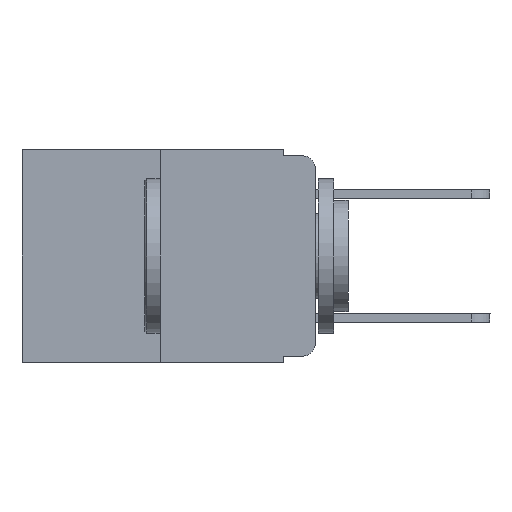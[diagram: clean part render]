
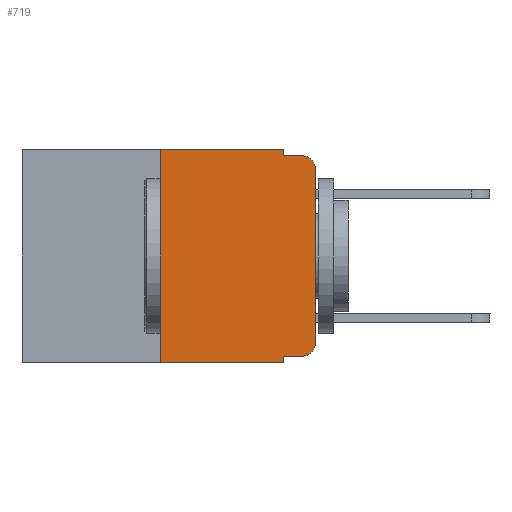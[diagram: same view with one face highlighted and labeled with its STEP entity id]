
A CAD part, left-side view. The second image highlights one B-rep face of the part: STEP entity #719.
In plain terms, the highlighted planar face has unit normal (-1, 0, 0).
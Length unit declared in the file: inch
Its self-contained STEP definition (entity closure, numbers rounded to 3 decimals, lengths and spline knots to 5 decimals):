
#53 = DIRECTION ( 'NONE',  ( 0., -1., 0. ) ) ;
#336 = ORIENTED_EDGE ( 'NONE', *, *, #405, .T. ) ;
#405 = EDGE_CURVE ( 'NONE', #3008, #11672, #10132, .T. ) ;
#460 = DIRECTION ( 'NONE',  ( 1., 0., 0. ) ) ;
#622 = LINE ( 'NONE', #12694, #4878 ) ;
#719 = ADVANCED_FACE ( 'NONE', ( #5134 ), #4983, .F. ) ;
#853 = EDGE_LOOP ( 'NONE', ( #336, #5707, #4773, #11057, #8538, #11031, #7886, #1759, #9447, #5569 ) ) ;
#878 = LINE ( 'NONE', #13318, #14174 ) ;
#914 = CARTESIAN_POINT ( 'NONE',  ( 0., 0.25, -0.343 ) ) ;
#939 = EDGE_CURVE ( 'NONE', #11672, #1989, #8153, .T. ) ;
#1031 = CARTESIAN_POINT ( 'NONE',  ( 0., 0.02, -0.01 ) ) ;
#1291 = CARTESIAN_POINT ( 'NONE',  ( 0., 0.473, -0.343 ) ) ;
#1348 = DIRECTION ( 'NONE',  ( 0., 0., -1. ) ) ;
#1683 = CARTESIAN_POINT ( 'NONE',  ( 0., 0., 0. ) ) ;
#1759 = ORIENTED_EDGE ( 'NONE', *, *, #8592, .F. ) ;
#1989 = VERTEX_POINT ( 'NONE', #1031 ) ;
#2348 = CARTESIAN_POINT ( 'NONE',  ( 0., 0.051, -0.333 ) ) ;
#2366 = LINE ( 'NONE', #1291, #10726 ) ;
#2584 = CARTESIAN_POINT ( 'NONE',  ( 0., 0.051, 0. ) ) ;
#2849 = VERTEX_POINT ( 'NONE', #11474 ) ;
#3008 = VERTEX_POINT ( 'NONE', #6712 ) ;
#3200 = VERTEX_POINT ( 'NONE', #914 ) ;
#3328 = EDGE_CURVE ( 'NONE', #3200, #8352, #622, .T. ) ;
#3452 = LINE ( 'NONE', #9062, #9283 ) ;
#3486 = CARTESIAN_POINT ( 'NONE',  ( 0., 0.02, -0.313 ) ) ;
#3777 = EDGE_CURVE ( 'NONE', #6651, #10921, #3452, .T. ) ;
#3919 = VECTOR ( 'NONE', #11880, 39.37008 ) ;
#3969 = CARTESIAN_POINT ( 'NONE',  ( 0., 0.051, -0.333 ) ) ;
#3984 = AXIS2_PLACEMENT_3D ( 'NONE', #8078, #12652, #1348 ) ;
#4013 = CARTESIAN_POINT ( 'NONE',  ( 0., 0.25, 0. ) ) ;
#4122 = EDGE_CURVE ( 'NONE', #3200, #2849, #2366, .T. ) ;
#4135 = LINE ( 'NONE', #14390, #14038 ) ;
#4703 = CARTESIAN_POINT ( 'NONE',  ( 0., 0.02, -0.333 ) ) ;
#4773 = ORIENTED_EDGE ( 'NONE', *, *, #4932, .F. ) ;
#4878 = VECTOR ( 'NONE', #11605, 39.37008 ) ;
#4932 = EDGE_CURVE ( 'NONE', #10921, #1989, #13336, .T. ) ;
#4983 = PLANE ( 'NONE',  #9161 ) ;
#5134 = FACE_OUTER_BOUND ( 'NONE', #853, .T. ) ;
#5569 = ORIENTED_EDGE ( 'NONE', *, *, #6532, .T. ) ;
#5707 = ORIENTED_EDGE ( 'NONE', *, *, #939, .T. ) ;
#5766 = CARTESIAN_POINT ( 'NONE',  ( 0., 0.051, -0.01 ) ) ;
#6532 = EDGE_CURVE ( 'NONE', #8114, #3008, #14079, .T. ) ;
#6651 = VERTEX_POINT ( 'NONE', #2584 ) ;
#6712 = CARTESIAN_POINT ( 'NONE',  ( 0., 0., -0.313 ) ) ;
#6965 = DIRECTION ( 'NONE',  ( -1., 0., 0. ) ) ;
#7151 = VECTOR ( 'NONE', #11953, 39.37008 ) ;
#7259 = EDGE_CURVE ( 'NONE', #10892, #8114, #14594, .T. ) ;
#7886 = ORIENTED_EDGE ( 'NONE', *, *, #4122, .T. ) ;
#8078 = CARTESIAN_POINT ( 'NONE',  ( 0., 0.02, -0.03 ) ) ;
#8114 = VERTEX_POINT ( 'NONE', #4703 ) ;
#8153 = CIRCLE ( 'NONE', #3984, 0.02 ) ;
#8352 = VERTEX_POINT ( 'NONE', #4013 ) ;
#8538 = ORIENTED_EDGE ( 'NONE', *, *, #9924, .F. ) ;
#8592 = EDGE_CURVE ( 'NONE', #10892, #2849, #4135, .T. ) ;
#9062 = CARTESIAN_POINT ( 'NONE',  ( 0., 0.051, 0. ) ) ;
#9149 = CARTESIAN_POINT ( 'NONE',  ( 0., 0., -0.03 ) ) ;
#9161 = AXIS2_PLACEMENT_3D ( 'NONE', #12915, #460, #13947 ) ;
#9283 = VECTOR ( 'NONE', #12446, 39.37008 ) ;
#9447 = ORIENTED_EDGE ( 'NONE', *, *, #7259, .T. ) ;
#9924 = EDGE_CURVE ( 'NONE', #8352, #6651, #878, .T. ) ;
#9969 = DIRECTION ( 'NONE',  ( 0., -1., 0. ) ) ;
#10132 = LINE ( 'NONE', #1683, #3919 ) ;
#10670 = AXIS2_PLACEMENT_3D ( 'NONE', #3486, #6965, #11415 ) ;
#10726 = VECTOR ( 'NONE', #53, 39.37008 ) ;
#10764 = DIRECTION ( 'NONE',  ( 0., -1., 0. ) ) ;
#10892 = VERTEX_POINT ( 'NONE', #2348 ) ;
#10921 = VERTEX_POINT ( 'NONE', #5766 ) ;
#11031 = ORIENTED_EDGE ( 'NONE', *, *, #3328, .F. ) ;
#11057 = ORIENTED_EDGE ( 'NONE', *, *, #3777, .F. ) ;
#11415 = DIRECTION ( 'NONE',  ( 0., 0., -1. ) ) ;
#11474 = CARTESIAN_POINT ( 'NONE',  ( 0., 0.051, -0.343 ) ) ;
#11605 = DIRECTION ( 'NONE',  ( 0., 0., 1. ) ) ;
#11672 = VERTEX_POINT ( 'NONE', #9149 ) ;
#11880 = DIRECTION ( 'NONE',  ( 0., 0., 1. ) ) ;
#11953 = DIRECTION ( 'NONE',  ( 0., -1., 0. ) ) ;
#12446 = DIRECTION ( 'NONE',  ( 0., 0., -1. ) ) ;
#12652 = DIRECTION ( 'NONE',  ( -1., 0., 0. ) ) ;
#12694 = CARTESIAN_POINT ( 'NONE',  ( 0., 0.25, 0. ) ) ;
#12915 = CARTESIAN_POINT ( 'NONE',  ( 0., 0.473, 0. ) ) ;
#13029 = VECTOR ( 'NONE', #10764, 39.37008 ) ;
#13318 = CARTESIAN_POINT ( 'NONE',  ( 0., 0.473, 0. ) ) ;
#13336 = LINE ( 'NONE', #14110, #7151 ) ;
#13947 = DIRECTION ( 'NONE',  ( 0., 0., -1. ) ) ;
#14038 = VECTOR ( 'NONE', #14057, 39.37008 ) ;
#14057 = DIRECTION ( 'NONE',  ( 0., 0., -1. ) ) ;
#14079 = CIRCLE ( 'NONE', #10670, 0.02 ) ;
#14110 = CARTESIAN_POINT ( 'NONE',  ( 0., 0.051, -0.01 ) ) ;
#14174 = VECTOR ( 'NONE', #9969, 39.37008 ) ;
#14390 = CARTESIAN_POINT ( 'NONE',  ( 0., 0.051, 0. ) ) ;
#14594 = LINE ( 'NONE', #3969, #13029 ) ;
